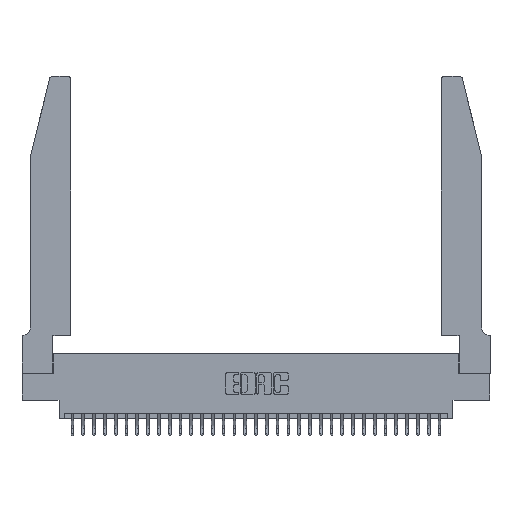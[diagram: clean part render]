
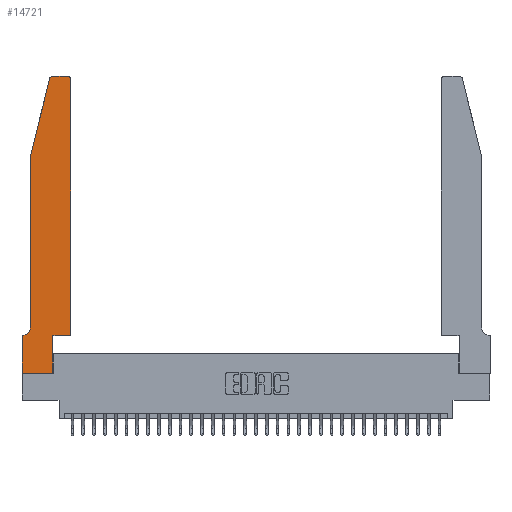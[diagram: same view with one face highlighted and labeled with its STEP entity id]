
A CAD part, top view. The second image highlights one B-rep face of the part: STEP entity #14721.
In plain terms, the highlighted planar face has unit normal (0, 0, 1).
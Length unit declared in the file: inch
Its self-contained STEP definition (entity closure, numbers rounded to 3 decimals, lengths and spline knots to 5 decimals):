
#468 = EDGE_CURVE ( 'NONE', #15935, #1871, #2039, .T. ) ;
#993 = EDGE_CURVE ( 'NONE', #28516, #30158, #25296, .T. ) ;
#1071 = ORIENTED_EDGE ( 'NONE', *, *, #468, .T. ) ;
#1287 = CARTESIAN_POINT ( 'NONE',  ( 0.0755, 0.42, 0.37 ) ) ;
#1871 = VERTEX_POINT ( 'NONE', #27883 ) ;
#2039 = CIRCLE ( 'NONE', #26015, 0.07 ) ;
#2630 = DIRECTION ( 'NONE',  ( -1., 0., 0. ) ) ;
#2646 = AXIS2_PLACEMENT_3D ( 'NONE', #12647, #30746, #28473 ) ;
#2956 = CARTESIAN_POINT ( 'NONE',  ( 0.0755, 2., 0.37 ) ) ;
#3161 = EDGE_CURVE ( 'NONE', #14524, #26646, #11811, .T. ) ;
#3596 = CARTESIAN_POINT ( 'NONE',  ( 0., 0.35, 0.37 ) ) ;
#3887 = AXIS2_PLACEMENT_3D ( 'NONE', #3596, #26809, #5982 ) ;
#4118 = EDGE_CURVE ( 'NONE', #26646, #18500, #30380, .T. ) ;
#4543 = EDGE_CURVE ( 'NONE', #11154, #14524, #33188, .T. ) ;
#4781 = VECTOR ( 'NONE', #23556, 39.37008 ) ;
#4796 = DIRECTION ( 'NONE',  ( -0.239, -0.971, 0. ) ) ;
#5412 = CARTESIAN_POINT ( 'NONE',  ( 0.2865, 0., 0.37 ) ) ;
#5835 = LINE ( 'NONE', #10805, #27329 ) ;
#5982 = DIRECTION ( 'NONE',  ( 1., 0., 0. ) ) ;
#6240 = EDGE_CURVE ( 'NONE', #24949, #15935, #10820, .T. ) ;
#6662 = FACE_OUTER_BOUND ( 'NONE', #31502, .T. ) ;
#6669 = EDGE_CURVE ( 'NONE', #30158, #28232, #13245, .T. ) ;
#6948 = CARTESIAN_POINT ( 'NONE',  ( 0.2865, 0.35, 0.37 ) ) ;
#7026 = LINE ( 'NONE', #7632, #11472 ) ;
#7632 = CARTESIAN_POINT ( 'NONE',  ( 0.0755, 2., 0.37 ) ) ;
#7968 = CARTESIAN_POINT ( 'NONE',  ( 0.0055, 0.42, 0.37 ) ) ;
#8153 = ORIENTED_EDGE ( 'NONE', *, *, #13910, .T. ) ;
#10287 = DIRECTION ( 'NONE',  ( 1., 0., 0. ) ) ;
#10805 = CARTESIAN_POINT ( 'NONE',  ( 0., 0., 0.37 ) ) ;
#10820 = LINE ( 'NONE', #2956, #23779 ) ;
#11064 = PLANE ( 'NONE',  #3887 ) ;
#11154 = VERTEX_POINT ( 'NONE', #33401 ) ;
#11472 = VECTOR ( 'NONE', #4796, 39.37008 ) ;
#11689 = CARTESIAN_POINT ( 'NONE',  ( 0., 0.35, 0.37 ) ) ;
#11811 = LINE ( 'NONE', #16702, #29627 ) ;
#12647 = CARTESIAN_POINT ( 'NONE',  ( 0.284, 2.72, 0.37 ) ) ;
#12699 = CARTESIAN_POINT ( 'NONE',  ( 0., 0., 0.37 ) ) ;
#13245 = LINE ( 'NONE', #6948, #33091 ) ;
#13354 = CARTESIAN_POINT ( 'NONE',  ( 0.4205, 2.75, 0.37 ) ) ;
#13412 = VERTEX_POINT ( 'NONE', #15439 ) ;
#13779 = LINE ( 'NONE', #20772, #32806 ) ;
#13829 = DIRECTION ( 'NONE',  ( 0., 0., 1. ) ) ;
#13893 = DIRECTION ( 'NONE',  ( 0., -1., 0. ) ) ;
#13910 = EDGE_CURVE ( 'NONE', #28232, #13412, #30700, .T. ) ;
#13917 = ORIENTED_EDGE ( 'NONE', *, *, #30902, .T. ) ;
#14417 = ORIENTED_EDGE ( 'NONE', *, *, #6669, .T. ) ;
#14498 = ORIENTED_EDGE ( 'NONE', *, *, #4118, .T. ) ;
#14524 = VERTEX_POINT ( 'NONE', #13354 ) ;
#14635 = ORIENTED_EDGE ( 'NONE', *, *, #4543, .T. ) ;
#14636 = LINE ( 'NONE', #17421, #21868 ) ;
#14716 = ORIENTED_EDGE ( 'NONE', *, *, #16632, .T. ) ;
#14721 = ADVANCED_FACE ( 'NONE', ( #6662 ), #11064, .T. ) ;
#15439 = CARTESIAN_POINT ( 'NONE',  ( 0.4505, 0.35, 0.37 ) ) ;
#15935 = VERTEX_POINT ( 'NONE', #1287 ) ;
#16435 = DIRECTION ( 'NONE',  ( 1., 0., 0. ) ) ;
#16632 = EDGE_CURVE ( 'NONE', #1871, #17744, #14636, .T. ) ;
#16702 = CARTESIAN_POINT ( 'NONE',  ( 0.2605, 2.75, 0.37 ) ) ;
#17407 = CARTESIAN_POINT ( 'NONE',  ( 0.2865, 0.35, 0.37 ) ) ;
#17421 = CARTESIAN_POINT ( 'NONE',  ( 0.0755, 0.35, 0.37 ) ) ;
#17744 = VERTEX_POINT ( 'NONE', #11689 ) ;
#18327 = ORIENTED_EDGE ( 'NONE', *, *, #993, .T. ) ;
#18500 = VERTEX_POINT ( 'NONE', #31383 ) ;
#19519 = ORIENTED_EDGE ( 'NONE', *, *, #31373, .T. ) ;
#20772 = CARTESIAN_POINT ( 'NONE',  ( 0.4505, 0.35, 0.37 ) ) ;
#20837 = CARTESIAN_POINT ( 'NONE',  ( 0., 0., 0.37 ) ) ;
#21398 = CARTESIAN_POINT ( 'NONE',  ( 0.284, 2.75, 0.37 ) ) ;
#21868 = VECTOR ( 'NONE', #32444, 39.37008 ) ;
#22879 = EDGE_CURVE ( 'NONE', #13412, #11154, #13779, .T. ) ;
#23284 = VECTOR ( 'NONE', #10287, 39.37008 ) ;
#23556 = DIRECTION ( 'NONE',  ( 1., 0., 0. ) ) ;
#23779 = VECTOR ( 'NONE', #24086, 39.37008 ) ;
#24086 = DIRECTION ( 'NONE',  ( 0., -1., 0. ) ) ;
#24090 = CARTESIAN_POINT ( 'NONE',  ( 0.4205, 2.72, 0.37 ) ) ;
#24129 = AXIS2_PLACEMENT_3D ( 'NONE', #24090, #13829, #16435 ) ;
#24949 = VERTEX_POINT ( 'NONE', #27185 ) ;
#25296 = LINE ( 'NONE', #12699, #23284 ) ;
#25638 = DIRECTION ( 'NONE',  ( 0., 1., 0. ) ) ;
#26015 = AXIS2_PLACEMENT_3D ( 'NONE', #7968, #28686, #2630 ) ;
#26646 = VERTEX_POINT ( 'NONE', #21398 ) ;
#26809 = DIRECTION ( 'NONE',  ( 0., 0., 1. ) ) ;
#26862 = DIRECTION ( 'NONE',  ( -1., 0., 0. ) ) ;
#27185 = CARTESIAN_POINT ( 'NONE',  ( 0.0755, 2., 0.37 ) ) ;
#27329 = VECTOR ( 'NONE', #13893, 39.37008 ) ;
#27883 = CARTESIAN_POINT ( 'NONE',  ( 0.0055, 0.35, 0.37 ) ) ;
#28232 = VERTEX_POINT ( 'NONE', #17407 ) ;
#28473 = DIRECTION ( 'NONE',  ( 1., 0., 0. ) ) ;
#28516 = VERTEX_POINT ( 'NONE', #20837 ) ;
#28686 = DIRECTION ( 'NONE',  ( 0., 0., -1. ) ) ;
#28993 = CARTESIAN_POINT ( 'NONE',  ( 0.4505, 0.35, 0.37 ) ) ;
#29046 = ORIENTED_EDGE ( 'NONE', *, *, #22879, .T. ) ;
#29627 = VECTOR ( 'NONE', #26862, 39.37008 ) ;
#30158 = VERTEX_POINT ( 'NONE', #5412 ) ;
#30380 = CIRCLE ( 'NONE', #2646, 0.03 ) ;
#30700 = LINE ( 'NONE', #28993, #4781 ) ;
#30746 = DIRECTION ( 'NONE',  ( 0., 0., 1. ) ) ;
#30902 = EDGE_CURVE ( 'NONE', #17744, #28516, #5835, .T. ) ;
#31373 = EDGE_CURVE ( 'NONE', #18500, #24949, #7026, .T. ) ;
#31383 = CARTESIAN_POINT ( 'NONE',  ( 0.25487, 2.72718, 0.37 ) ) ;
#31502 = EDGE_LOOP ( 'NONE', ( #32688, #14498, #19519, #33199, #1071, #14716, #13917, #18327, #14417, #8153, #29046, #14635 ) ) ;
#32444 = DIRECTION ( 'NONE',  ( -1., 0., 0. ) ) ;
#32688 = ORIENTED_EDGE ( 'NONE', *, *, #3161, .T. ) ;
#32806 = VECTOR ( 'NONE', #25638, 39.37008 ) ;
#32884 = DIRECTION ( 'NONE',  ( 0., 1., 0. ) ) ;
#33091 = VECTOR ( 'NONE', #32884, 39.37008 ) ;
#33188 = CIRCLE ( 'NONE', #24129, 0.03 ) ;
#33199 = ORIENTED_EDGE ( 'NONE', *, *, #6240, .T. ) ;
#33401 = CARTESIAN_POINT ( 'NONE',  ( 0.4505, 2.72, 0.37 ) ) ;
